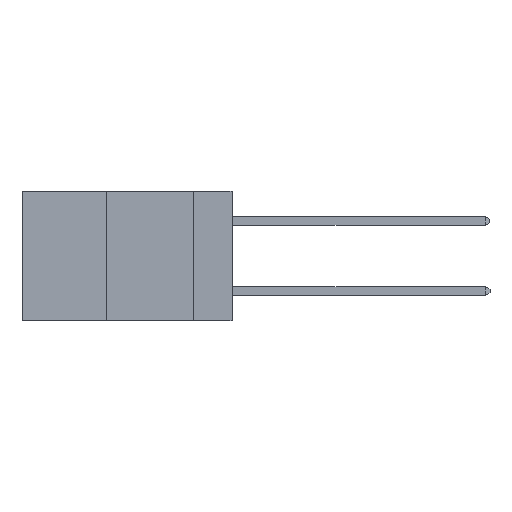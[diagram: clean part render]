
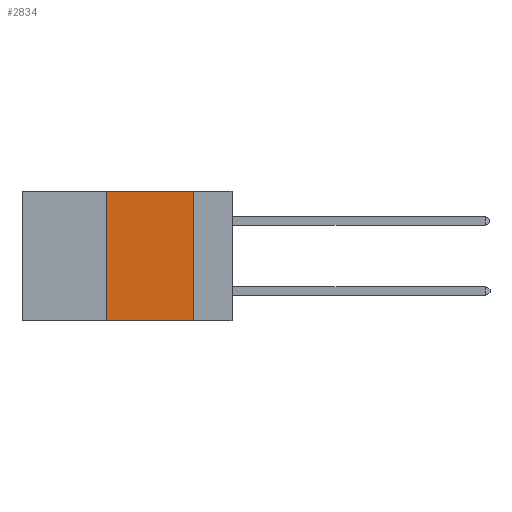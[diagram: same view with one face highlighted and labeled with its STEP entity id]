
A CAD part, left-side view. The second image highlights one B-rep face of the part: STEP entity #2834.
In plain terms, the highlighted planar face has unit normal (-1, 0, 0).
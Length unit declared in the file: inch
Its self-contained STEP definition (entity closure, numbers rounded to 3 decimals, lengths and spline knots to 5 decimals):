
#884 = VECTOR ( 'NONE', #13444, 39.37008 ) ;
#969 = VERTEX_POINT ( 'NONE', #8657 ) ;
#2803 = EDGE_LOOP ( 'NONE', ( #8283, #12202, #8751, #16619 ) ) ;
#2834 = ADVANCED_FACE ( 'NONE', ( #18538 ), #13607, .F. ) ;
#2919 = VECTOR ( 'NONE', #8247, 39.37008 ) ;
#3049 = CARTESIAN_POINT ( 'NONE',  ( 0., 0.36, 0. ) ) ;
#3935 = CARTESIAN_POINT ( 'NONE',  ( 0., 0.36, -0.37 ) ) ;
#4699 = DIRECTION ( 'NONE',  ( 1., 0., 0. ) ) ;
#5285 = EDGE_CURVE ( 'NONE', #5723, #8181, #9546, .T. ) ;
#5368 = EDGE_CURVE ( 'NONE', #969, #5723, #11619, .T. ) ;
#5723 = VERTEX_POINT ( 'NONE', #18513 ) ;
#5781 = DIRECTION ( 'NONE',  ( 0., -1., 0. ) ) ;
#5931 = EDGE_CURVE ( 'NONE', #7521, #969, #12297, .T. ) ;
#7231 = CARTESIAN_POINT ( 'NONE',  ( 0., 0.11, -0.37 ) ) ;
#7302 = CARTESIAN_POINT ( 'NONE',  ( 0., 0.6, 0. ) ) ;
#7521 = VERTEX_POINT ( 'NONE', #3935 ) ;
#8181 = VERTEX_POINT ( 'NONE', #7231 ) ;
#8247 = DIRECTION ( 'NONE',  ( 0., -1., 0. ) ) ;
#8283 = ORIENTED_EDGE ( 'NONE', *, *, #5285, .F. ) ;
#8657 = CARTESIAN_POINT ( 'NONE',  ( 0., 0.36, 0. ) ) ;
#8673 = EDGE_CURVE ( 'NONE', #7521, #8181, #18657, .T. ) ;
#8751 = ORIENTED_EDGE ( 'NONE', *, *, #5931, .F. ) ;
#9546 = LINE ( 'NONE', #14499, #13952 ) ;
#11619 = LINE ( 'NONE', #7302, #18970 ) ;
#12091 = CARTESIAN_POINT ( 'NONE',  ( 0., 0.6, 0. ) ) ;
#12202 = ORIENTED_EDGE ( 'NONE', *, *, #5368, .F. ) ;
#12297 = LINE ( 'NONE', #3049, #884 ) ;
#13444 = DIRECTION ( 'NONE',  ( 0., 0., 1. ) ) ;
#13607 = PLANE ( 'NONE',  #16637 ) ;
#13952 = VECTOR ( 'NONE', #16001, 39.37008 ) ;
#14153 = CARTESIAN_POINT ( 'NONE',  ( 0., 0.6, -0.37 ) ) ;
#14499 = CARTESIAN_POINT ( 'NONE',  ( 0., 0.11, 0. ) ) ;
#15096 = DIRECTION ( 'NONE',  ( 0., 0., -1. ) ) ;
#16001 = DIRECTION ( 'NONE',  ( 0., 0., -1. ) ) ;
#16619 = ORIENTED_EDGE ( 'NONE', *, *, #8673, .T. ) ;
#16637 = AXIS2_PLACEMENT_3D ( 'NONE', #12091, #4699, #15096 ) ;
#18513 = CARTESIAN_POINT ( 'NONE',  ( 0., 0.11, 0. ) ) ;
#18538 = FACE_OUTER_BOUND ( 'NONE', #2803, .T. ) ;
#18657 = LINE ( 'NONE', #14153, #2919 ) ;
#18970 = VECTOR ( 'NONE', #5781, 39.37008 ) ;
